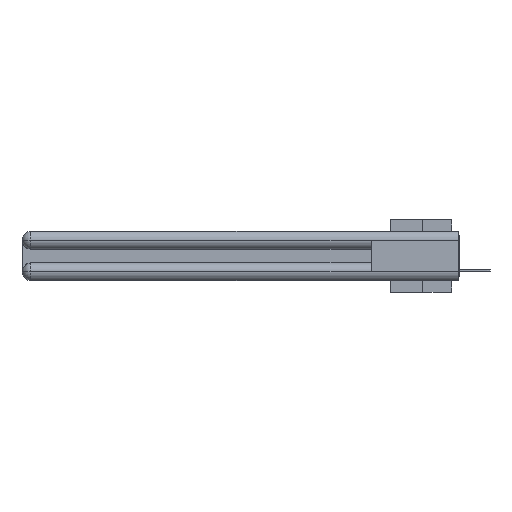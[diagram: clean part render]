
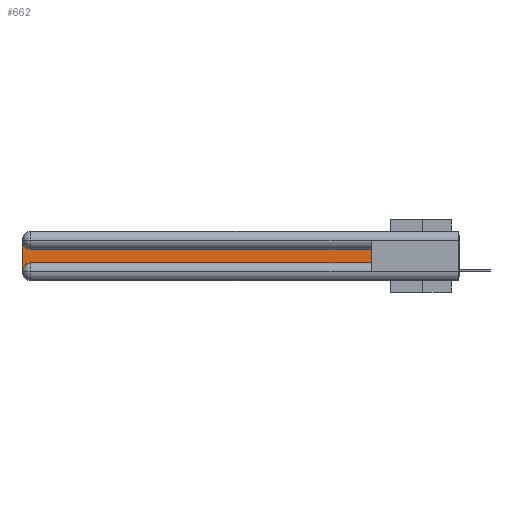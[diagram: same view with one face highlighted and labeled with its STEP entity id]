
A CAD part, left-side view. The second image highlights one B-rep face of the part: STEP entity #662.
In plain terms, the highlighted planar face has unit normal (-1, 0, 0).
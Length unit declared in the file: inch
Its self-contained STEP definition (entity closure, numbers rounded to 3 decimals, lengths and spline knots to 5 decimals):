
#47 = VERTEX_POINT ( 'NONE', #36897 ) ;
#662 = ADVANCED_FACE ( 'NONE', ( #8555 ), #32464, .F. ) ;
#723 = CIRCLE ( 'NONE', #17257, 0.06 ) ;
#900 = EDGE_CURVE ( 'NONE', #5004, #27279, #18149, .T. ) ;
#1380 = LINE ( 'NONE', #23045, #12715 ) ;
#2986 = DIRECTION ( 'NONE',  ( 0., 0., 1. ) ) ;
#3763 = VECTOR ( 'NONE', #2986, 39.37008 ) ;
#4080 = ORIENTED_EDGE ( 'NONE', *, *, #900, .T. ) ;
#4737 = CARTESIAN_POINT ( 'NONE',  ( 0.075, 0.6, -0.2175 ) ) ;
#5004 = VERTEX_POINT ( 'NONE', #14295 ) ;
#6850 = CARTESIAN_POINT ( 'NONE',  ( 0.075, 2.94, -0.0625 ) ) ;
#7553 = DIRECTION ( 'NONE',  ( 1., 0., 0. ) ) ;
#8555 = FACE_OUTER_BOUND ( 'NONE', #8825, .T. ) ;
#8825 = EDGE_LOOP ( 'NONE', ( #4080, #21831, #26060, #10918, #20091, #9674 ) ) ;
#9674 = ORIENTED_EDGE ( 'NONE', *, *, #31966, .T. ) ;
#10176 = DIRECTION ( 'NONE',  ( 0., 1., 0. ) ) ;
#10918 = ORIENTED_EDGE ( 'NONE', *, *, #15658, .T. ) ;
#11704 = VERTEX_POINT ( 'NONE', #25506 ) ;
#12715 = VECTOR ( 'NONE', #20136, 39.37008 ) ;
#13129 = DIRECTION ( 'NONE',  ( 1., 0., 0. ) ) ;
#14254 = VECTOR ( 'NONE', #10176, 39.37008 ) ;
#14295 = CARTESIAN_POINT ( 'NONE',  ( 0.075, 0.6, -0.1225 ) ) ;
#14809 = VERTEX_POINT ( 'NONE', #27501 ) ;
#15658 = EDGE_CURVE ( 'NONE', #47, #21972, #29859, .T. ) ;
#16758 = DIRECTION ( 'NONE',  ( 1., 0., 0. ) ) ;
#17257 = AXIS2_PLACEMENT_3D ( 'NONE', #6850, #13129, #35009 ) ;
#17487 = AXIS2_PLACEMENT_3D ( 'NONE', #19420, #7553, #22754 ) ;
#18149 = LINE ( 'NONE', #31669, #14254 ) ;
#19420 = CARTESIAN_POINT ( 'NONE',  ( 0.075, 2.94, -0.2775 ) ) ;
#20091 = ORIENTED_EDGE ( 'NONE', *, *, #35817, .T. ) ;
#20136 = DIRECTION ( 'NONE',  ( 0., 0., -1. ) ) ;
#21831 = ORIENTED_EDGE ( 'NONE', *, *, #36740, .T. ) ;
#21972 = VERTEX_POINT ( 'NONE', #23112 ) ;
#22754 = DIRECTION ( 'NONE',  ( 0., 0., -1. ) ) ;
#23045 = CARTESIAN_POINT ( 'NONE',  ( 0.075, 3., -0.2175 ) ) ;
#23112 = CARTESIAN_POINT ( 'NONE',  ( 0.075, 2.94, -0.2175 ) ) ;
#25506 = CARTESIAN_POINT ( 'NONE',  ( 0.075, 0.6, -0.2175 ) ) ;
#26060 = ORIENTED_EDGE ( 'NONE', *, *, #39578, .T. ) ;
#26402 = DIRECTION ( 'NONE',  ( 0., -1., 0. ) ) ;
#27279 = VERTEX_POINT ( 'NONE', #31069 ) ;
#27501 = CARTESIAN_POINT ( 'NONE',  ( 0.075, 3., -0.0625 ) ) ;
#29859 = CIRCLE ( 'NONE', #17487, 0.06 ) ;
#31069 = CARTESIAN_POINT ( 'NONE',  ( 0.075, 2.94, -0.1225 ) ) ;
#31669 = CARTESIAN_POINT ( 'NONE',  ( 0.075, 0.6, -0.1225 ) ) ;
#31966 = EDGE_CURVE ( 'NONE', #11704, #5004, #36829, .T. ) ;
#32464 = PLANE ( 'NONE',  #34942 ) ;
#34850 = LINE ( 'NONE', #4737, #40246 ) ;
#34942 = AXIS2_PLACEMENT_3D ( 'NONE', #35629, #16758, #38814 ) ;
#35009 = DIRECTION ( 'NONE',  ( 0., 0., -1. ) ) ;
#35629 = CARTESIAN_POINT ( 'NONE',  ( 0.075, 3., -0.1225 ) ) ;
#35817 = EDGE_CURVE ( 'NONE', #21972, #11704, #34850, .T. ) ;
#36740 = EDGE_CURVE ( 'NONE', #27279, #14809, #723, .T. ) ;
#36829 = LINE ( 'NONE', #40742, #3763 ) ;
#36897 = CARTESIAN_POINT ( 'NONE',  ( 0.075, 3., -0.2775 ) ) ;
#38814 = DIRECTION ( 'NONE',  ( 0., 0., -1. ) ) ;
#39578 = EDGE_CURVE ( 'NONE', #14809, #47, #1380, .T. ) ;
#40246 = VECTOR ( 'NONE', #26402, 39.37008 ) ;
#40742 = CARTESIAN_POINT ( 'NONE',  ( 0.075, 0.6, -0.2175 ) ) ;
